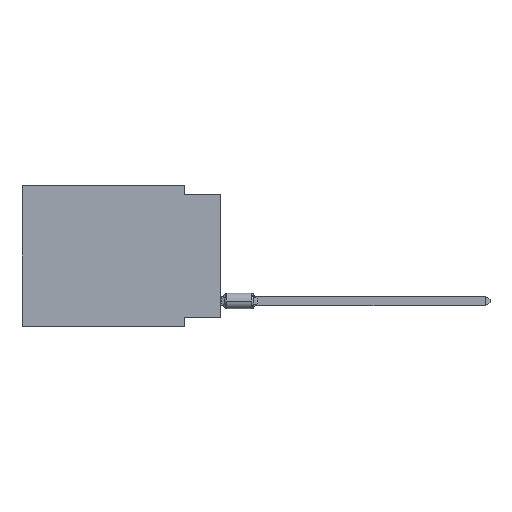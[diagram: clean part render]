
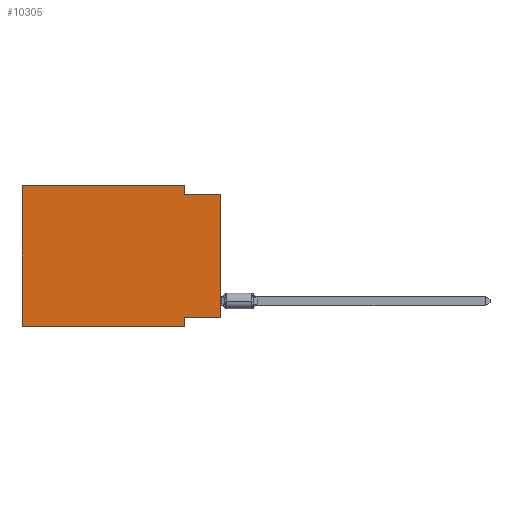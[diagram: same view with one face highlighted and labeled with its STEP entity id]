
A CAD part, left-side view. The second image highlights one B-rep face of the part: STEP entity #10305.
In plain terms, the highlighted planar face has unit normal (-1, 0, 0).
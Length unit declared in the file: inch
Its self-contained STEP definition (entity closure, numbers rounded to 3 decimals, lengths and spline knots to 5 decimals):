
#19 = CARTESIAN_POINT ( 'NONE',  ( 0., 0.1, -0.365 ) ) ;
#171 = LINE ( 'NONE', #1352, #5089 ) ;
#428 = CARTESIAN_POINT ( 'NONE',  ( 0., 0.1, -0.025 ) ) ;
#708 = EDGE_CURVE ( 'NONE', #8317, #8661, #747, .T. ) ;
#747 = LINE ( 'NONE', #15059, #2391 ) ;
#1040 = VERTEX_POINT ( 'NONE', #12823 ) ;
#1146 = ORIENTED_EDGE ( 'NONE', *, *, #13005, .F. ) ;
#1295 = VECTOR ( 'NONE', #11503, 39.37008 ) ;
#1352 = CARTESIAN_POINT ( 'NONE',  ( 0., 0., 0. ) ) ;
#1480 = FACE_OUTER_BOUND ( 'NONE', #5124, .T. ) ;
#1985 = VERTEX_POINT ( 'NONE', #6178 ) ;
#2026 = DIRECTION ( 'NONE',  ( 0., -1., 0. ) ) ;
#2391 = VECTOR ( 'NONE', #12695, 39.37008 ) ;
#2577 = VECTOR ( 'NONE', #4691, 39.37008 ) ;
#3778 = VECTOR ( 'NONE', #8771, 39.37008 ) ;
#3976 = CARTESIAN_POINT ( 'NONE',  ( 0., 0., -0.025 ) ) ;
#4691 = DIRECTION ( 'NONE',  ( 0., 0., -1. ) ) ;
#4739 = VECTOR ( 'NONE', #13206, 39.37008 ) ;
#4933 = LINE ( 'NONE', #7212, #6996 ) ;
#4954 = PLANE ( 'NONE',  #8336 ) ;
#5089 = VECTOR ( 'NONE', #8355, 39.37008 ) ;
#5124 = EDGE_LOOP ( 'NONE', ( #8550, #7437, #7045, #5826, #11255, #8218, #1146, #7597 ) ) ;
#5399 = VERTEX_POINT ( 'NONE', #428 ) ;
#5622 = CARTESIAN_POINT ( 'NONE',  ( 0., 0.1, 0. ) ) ;
#5826 = ORIENTED_EDGE ( 'NONE', *, *, #7223, .F. ) ;
#5876 = LINE ( 'NONE', #15465, #2577 ) ;
#6028 = DIRECTION ( 'NONE',  ( 0., 0., 1. ) ) ;
#6178 = CARTESIAN_POINT ( 'NONE',  ( 0., 0., -0.025 ) ) ;
#6335 = CARTESIAN_POINT ( 'NONE',  ( 0., 0.1, -0.39 ) ) ;
#6436 = VERTEX_POINT ( 'NONE', #6335 ) ;
#6507 = EDGE_CURVE ( 'NONE', #14030, #1040, #4933, .T. ) ;
#6996 = VECTOR ( 'NONE', #6028, 39.37008 ) ;
#7045 = ORIENTED_EDGE ( 'NONE', *, *, #12071, .F. ) ;
#7078 = VECTOR ( 'NONE', #2026, 39.37008 ) ;
#7212 = CARTESIAN_POINT ( 'NONE',  ( 0., 0.55, 0. ) ) ;
#7223 = EDGE_CURVE ( 'NONE', #1040, #12454, #12186, .T. ) ;
#7397 = DIRECTION ( 'NONE',  ( 0., 0., -1. ) ) ;
#7437 = ORIENTED_EDGE ( 'NONE', *, *, #9182, .F. ) ;
#7597 = ORIENTED_EDGE ( 'NONE', *, *, #708, .F. ) ;
#8218 = ORIENTED_EDGE ( 'NONE', *, *, #10522, .T. ) ;
#8294 = CARTESIAN_POINT ( 'NONE',  ( 0., 0., -0.365 ) ) ;
#8317 = VERTEX_POINT ( 'NONE', #8294 ) ;
#8336 = AXIS2_PLACEMENT_3D ( 'NONE', #8563, #12105, #7397 ) ;
#8355 = DIRECTION ( 'NONE',  ( 0., 0., 1. ) ) ;
#8429 = CARTESIAN_POINT ( 'NONE',  ( 0., 0.55, 0. ) ) ;
#8550 = ORIENTED_EDGE ( 'NONE', *, *, #15397, .T. ) ;
#8563 = CARTESIAN_POINT ( 'NONE',  ( 0., 0.55, 0. ) ) ;
#8661 = VERTEX_POINT ( 'NONE', #19 ) ;
#8771 = DIRECTION ( 'NONE',  ( 0., -1., 0. ) ) ;
#9070 = LINE ( 'NONE', #5622, #1295 ) ;
#9182 = EDGE_CURVE ( 'NONE', #5399, #1985, #14749, .T. ) ;
#10305 = ADVANCED_FACE ( 'NONE', ( #1480 ), #4954, .F. ) ;
#10522 = EDGE_CURVE ( 'NONE', #14030, #6436, #11455, .T. ) ;
#11255 = ORIENTED_EDGE ( 'NONE', *, *, #6507, .F. ) ;
#11455 = LINE ( 'NONE', #13964, #7078 ) ;
#11503 = DIRECTION ( 'NONE',  ( 0., 0., -1. ) ) ;
#12071 = EDGE_CURVE ( 'NONE', #12454, #5399, #9070, .T. ) ;
#12105 = DIRECTION ( 'NONE',  ( 1., 0., 0. ) ) ;
#12186 = LINE ( 'NONE', #8429, #4739 ) ;
#12454 = VERTEX_POINT ( 'NONE', #14797 ) ;
#12695 = DIRECTION ( 'NONE',  ( 0., 1., 0. ) ) ;
#12823 = CARTESIAN_POINT ( 'NONE',  ( 0., 0.55, 0. ) ) ;
#12957 = CARTESIAN_POINT ( 'NONE',  ( 0., 0.55, -0.39 ) ) ;
#13005 = EDGE_CURVE ( 'NONE', #8661, #6436, #5876, .T. ) ;
#13206 = DIRECTION ( 'NONE',  ( 0., -1., 0. ) ) ;
#13964 = CARTESIAN_POINT ( 'NONE',  ( 0., 0.55, -0.39 ) ) ;
#14030 = VERTEX_POINT ( 'NONE', #12957 ) ;
#14749 = LINE ( 'NONE', #3976, #3778 ) ;
#14797 = CARTESIAN_POINT ( 'NONE',  ( 0., 0.1, 0. ) ) ;
#15059 = CARTESIAN_POINT ( 'NONE',  ( 0., 0., -0.365 ) ) ;
#15397 = EDGE_CURVE ( 'NONE', #8317, #1985, #171, .T. ) ;
#15465 = CARTESIAN_POINT ( 'NONE',  ( 0., 0.1, -0.39 ) ) ;
